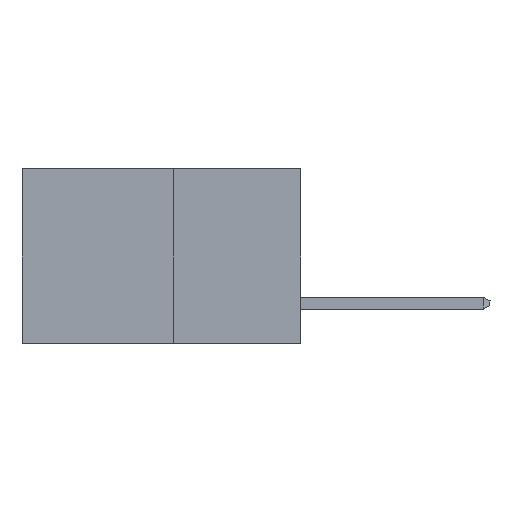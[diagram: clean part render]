
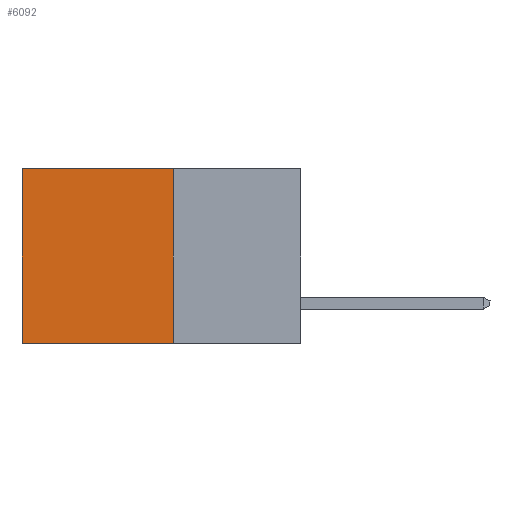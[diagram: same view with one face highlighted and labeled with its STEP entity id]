
A CAD part, left-side view. The second image highlights one B-rep face of the part: STEP entity #6092.
In plain terms, the highlighted planar face has unit normal (-1, 0, 0).
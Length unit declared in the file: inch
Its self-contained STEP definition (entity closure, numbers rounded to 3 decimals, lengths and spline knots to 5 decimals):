
#403 = ORIENTED_EDGE ( 'NONE', *, *, #7937, .T. ) ;
#422 = FACE_OUTER_BOUND ( 'NONE', #8260, .T. ) ;
#868 = ORIENTED_EDGE ( 'NONE', *, *, #7147, .F. ) ;
#1015 = DIRECTION ( 'NONE',  ( 0., 1., 0. ) ) ;
#1025 = DIRECTION ( 'NONE',  ( 0., 0., -1. ) ) ;
#1401 = EDGE_CURVE ( 'NONE', #9369, #7241, #3709, .T. ) ;
#1487 = VECTOR ( 'NONE', #4909, 39.37008 ) ;
#1610 = CARTESIAN_POINT ( 'NONE',  ( 0.277, 0.27, 0. ) ) ;
#1694 = DIRECTION ( 'NONE',  ( 0., 1., 0. ) ) ;
#2763 = VECTOR ( 'NONE', #1015, 39.37008 ) ;
#2901 = CARTESIAN_POINT ( 'NONE',  ( 0.277, 0.59, 0. ) ) ;
#3675 = VECTOR ( 'NONE', #1694, 39.37008 ) ;
#3700 = VERTEX_POINT ( 'NONE', #2901 ) ;
#3709 = LINE ( 'NONE', #7019, #1487 ) ;
#4510 = CARTESIAN_POINT ( 'NONE',  ( 0.277, 0.59, -0.37 ) ) ;
#4620 = ORIENTED_EDGE ( 'NONE', *, *, #1401, .F. ) ;
#4711 = LINE ( 'NONE', #5979, #2763 ) ;
#4752 = DIRECTION ( 'NONE',  ( 1., 0., 0. ) ) ;
#4831 = ORIENTED_EDGE ( 'NONE', *, *, #6038, .T. ) ;
#4848 = LINE ( 'NONE', #4510, #6518 ) ;
#4909 = DIRECTION ( 'NONE',  ( 0., 0., -1. ) ) ;
#5979 = CARTESIAN_POINT ( 'NONE',  ( 0.277, 0.27, -0.37 ) ) ;
#6027 = LINE ( 'NONE', #6496, #3675 ) ;
#6038 = EDGE_CURVE ( 'NONE', #3700, #7470, #4848, .T. ) ;
#6092 = ADVANCED_FACE ( 'NONE', ( #422 ), #7614, .F. ) ;
#6496 = CARTESIAN_POINT ( 'NONE',  ( 0.277, 0.27, 0. ) ) ;
#6518 = VECTOR ( 'NONE', #8786, 39.37008 ) ;
#6599 = AXIS2_PLACEMENT_3D ( 'NONE', #6868, #4752, #1025 ) ;
#6820 = CARTESIAN_POINT ( 'NONE',  ( 0.277, 0.59, -0.37 ) ) ;
#6868 = CARTESIAN_POINT ( 'NONE',  ( 0.277, 0.27, -0.37 ) ) ;
#7019 = CARTESIAN_POINT ( 'NONE',  ( 0.277, 0.27, -0.37 ) ) ;
#7147 = EDGE_CURVE ( 'NONE', #7241, #7470, #4711, .T. ) ;
#7241 = VERTEX_POINT ( 'NONE', #8689 ) ;
#7470 = VERTEX_POINT ( 'NONE', #6820 ) ;
#7614 = PLANE ( 'NONE',  #6599 ) ;
#7937 = EDGE_CURVE ( 'NONE', #9369, #3700, #6027, .T. ) ;
#8260 = EDGE_LOOP ( 'NONE', ( #4831, #868, #4620, #403 ) ) ;
#8689 = CARTESIAN_POINT ( 'NONE',  ( 0.277, 0.27, -0.37 ) ) ;
#8786 = DIRECTION ( 'NONE',  ( 0., 0., -1. ) ) ;
#9369 = VERTEX_POINT ( 'NONE', #1610 ) ;
